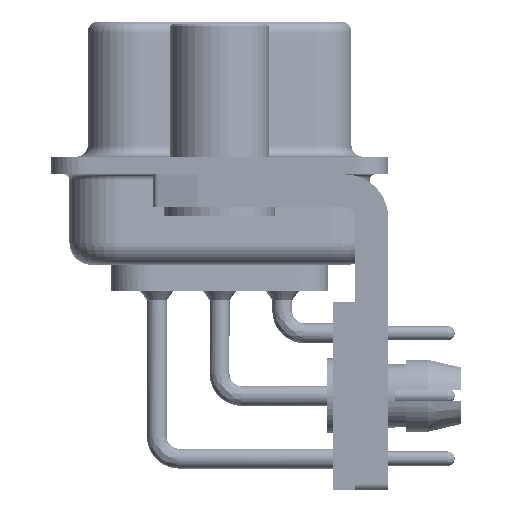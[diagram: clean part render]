
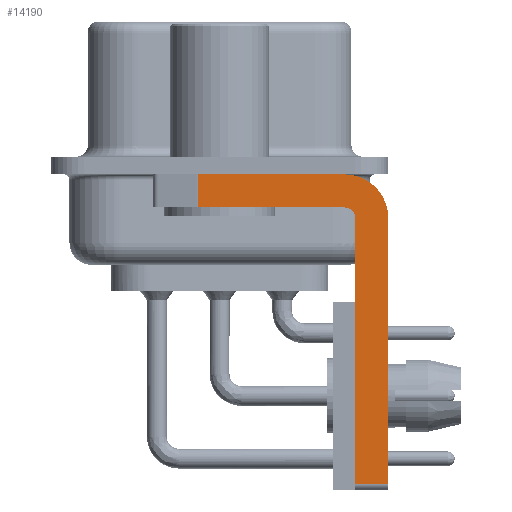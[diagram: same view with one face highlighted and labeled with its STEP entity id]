
A CAD part, left-side view. The second image highlights one B-rep face of the part: STEP entity #14190.
In plain terms, the highlighted planar face has unit normal (-1, 0, 0).
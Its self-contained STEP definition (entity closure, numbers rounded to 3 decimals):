
#886 = DIRECTION ( 'NONE',  ( 0., 1., 0. ) ) ;
#2552 = CARTESIAN_POINT ( 'NONE',  ( -2.9, -6.15, -14.45 ) ) ;
#3882 = LINE ( 'NONE', #14087, #38482 ) ;
#4366 = CARTESIAN_POINT ( 'NONE',  ( -2.9, -7.65, -14.45 ) ) ;
#4929 = CARTESIAN_POINT ( 'NONE',  ( -2.9, -7.65, -2.4 ) ) ;
#5027 = CARTESIAN_POINT ( 'NONE',  ( -2.9, -5.65, -2.4 ) ) ;
#5063 = DIRECTION ( 'NONE',  ( 1., 0., 0. ) ) ;
#7195 = DIRECTION ( 'NONE',  ( 0., -1., 0. ) ) ;
#7227 = DIRECTION ( 'NONE',  ( 0., -1., 0. ) ) ;
#8472 = DIRECTION ( 'NONE',  ( 0., 0., 1. ) ) ;
#9020 = CARTESIAN_POINT ( 'NONE',  ( -2.9, -6.15, -2.4 ) ) ;
#10486 = AXIS2_PLACEMENT_3D ( 'NONE', #43701, #40402, #19775 ) ;
#10743 = ORIENTED_EDGE ( 'NONE', *, *, #43785, .T. ) ;
#11012 = LINE ( 'NONE', #4929, #29444 ) ;
#12458 = ORIENTED_EDGE ( 'NONE', *, *, #40808, .F. ) ;
#13174 = VERTEX_POINT ( 'NONE', #32133 ) ;
#14087 = CARTESIAN_POINT ( 'NONE',  ( -2.9, -5.65, -14.45 ) ) ;
#14190 = ADVANCED_FACE ( 'NONE', ( #27897 ), #36943, .F. ) ;
#14226 = VECTOR ( 'NONE', #7195, 1000. ) ;
#14938 = EDGE_CURVE ( 'NONE', #41622, #30344, #38593, .T. ) ;
#16684 = DIRECTION ( 'NONE',  ( 0., 0., 1. ) ) ;
#17863 = VERTEX_POINT ( 'NONE', #20414 ) ;
#18114 = ORIENTED_EDGE ( 'NONE', *, *, #14938, .F. ) ;
#19775 = DIRECTION ( 'NONE',  ( 0., 0., -1. ) ) ;
#20382 = AXIS2_PLACEMENT_3D ( 'NONE', #5027, #29272, #8472 ) ;
#20414 = CARTESIAN_POINT ( 'NONE',  ( -2.9, -5.65, -0.4 ) ) ;
#20807 = VERTEX_POINT ( 'NONE', #4366 ) ;
#21230 = CARTESIAN_POINT ( 'NONE',  ( -2.9, -5.65, -1.9 ) ) ;
#21759 = CARTESIAN_POINT ( 'NONE',  ( -2.9, -5.65, -1.9 ) ) ;
#23322 = EDGE_LOOP ( 'NONE', ( #31443, #34856, #24407, #28069, #18114, #10743, #40978, #12458 ) ) ;
#23584 = CARTESIAN_POINT ( 'NONE',  ( -2.9, -7.65, -2.4 ) ) ;
#24407 = ORIENTED_EDGE ( 'NONE', *, *, #44544, .F. ) ;
#24539 = CARTESIAN_POINT ( 'NONE',  ( -2.9, 3., -0.4 ) ) ;
#25735 = DIRECTION ( 'NONE',  ( 0., 0., -1. ) ) ;
#25846 = CARTESIAN_POINT ( 'NONE',  ( -2.9, -5.65, -2.4 ) ) ;
#26442 = CIRCLE ( 'NONE', #20382, 0.5 ) ;
#26763 = CARTESIAN_POINT ( 'NONE',  ( -2.9, 0.978, -1.9 ) ) ;
#26909 = DIRECTION ( 'NONE',  ( 0., 0., -1. ) ) ;
#26989 = CARTESIAN_POINT ( 'NONE',  ( -2.9, -6.15, -14.7 ) ) ;
#27233 = VERTEX_POINT ( 'NONE', #21230 ) ;
#27897 = FACE_OUTER_BOUND ( 'NONE', #23322, .T. ) ;
#28069 = ORIENTED_EDGE ( 'NONE', *, *, #35783, .F. ) ;
#29272 = DIRECTION ( 'NONE',  ( -1., 0., 0. ) ) ;
#29308 = DIRECTION ( 'NONE',  ( 0., 0., -1. ) ) ;
#29444 = VECTOR ( 'NONE', #25735, 1000. ) ;
#29449 = VECTOR ( 'NONE', #16684, 1000. ) ;
#29587 = VERTEX_POINT ( 'NONE', #23584 ) ;
#30344 = VERTEX_POINT ( 'NONE', #9020 ) ;
#31279 = EDGE_CURVE ( 'NONE', #29587, #20807, #11012, .T. ) ;
#31443 = ORIENTED_EDGE ( 'NONE', *, *, #37061, .F. ) ;
#32133 = CARTESIAN_POINT ( 'NONE',  ( -2.9, 0.978, -0.4 ) ) ;
#32310 = CARTESIAN_POINT ( 'NONE',  ( -2.9, 0.978, -1.9 ) ) ;
#32377 = VECTOR ( 'NONE', #26909, 1000. ) ;
#32575 = LINE ( 'NONE', #24539, #14226 ) ;
#34856 = ORIENTED_EDGE ( 'NONE', *, *, #35355, .T. ) ;
#35355 = EDGE_CURVE ( 'NONE', #13174, #37220, #41521, .T. ) ;
#35783 = EDGE_CURVE ( 'NONE', #30344, #27233, #26442, .T. ) ;
#36943 = PLANE ( 'NONE',  #10486 ) ;
#37061 = EDGE_CURVE ( 'NONE', #13174, #17863, #32575, .T. ) ;
#37220 = VERTEX_POINT ( 'NONE', #32310 ) ;
#37842 = AXIS2_PLACEMENT_3D ( 'NONE', #25846, #5063, #29308 ) ;
#38482 = VECTOR ( 'NONE', #7227, 1000. ) ;
#38593 = LINE ( 'NONE', #26989, #29449 ) ;
#40026 = VECTOR ( 'NONE', #886, 1000. ) ;
#40402 = DIRECTION ( 'NONE',  ( 1., 0., 0. ) ) ;
#40808 = EDGE_CURVE ( 'NONE', #17863, #29587, #44149, .T. ) ;
#40978 = ORIENTED_EDGE ( 'NONE', *, *, #31279, .F. ) ;
#41521 = LINE ( 'NONE', #26763, #32377 ) ;
#41622 = VERTEX_POINT ( 'NONE', #2552 ) ;
#42184 = LINE ( 'NONE', #21759, #40026 ) ;
#43701 = CARTESIAN_POINT ( 'NONE',  ( -2.9, -5.65, -2.4 ) ) ;
#43785 = EDGE_CURVE ( 'NONE', #41622, #20807, #3882, .T. ) ;
#44149 = CIRCLE ( 'NONE', #37842, 2. ) ;
#44544 = EDGE_CURVE ( 'NONE', #27233, #37220, #42184, .T. ) ;
